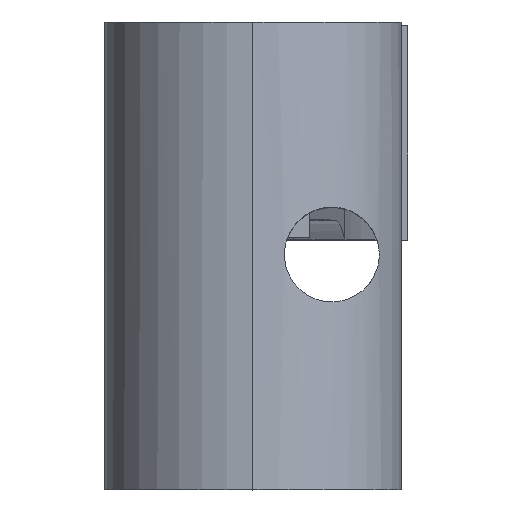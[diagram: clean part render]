
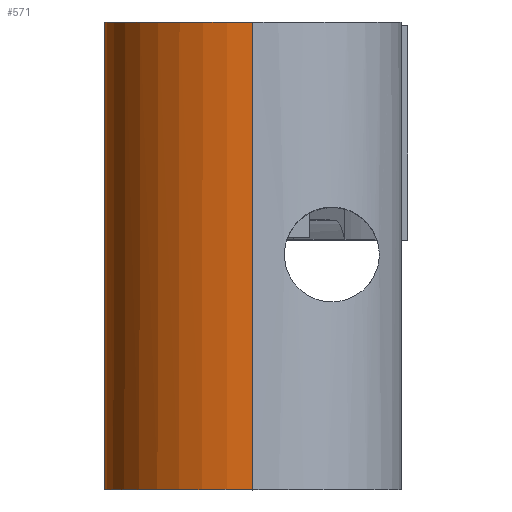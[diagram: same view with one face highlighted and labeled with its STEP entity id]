
A CAD part, top view. The second image highlights one B-rep face of the part: STEP entity #571.
In plain terms, the highlighted cylindrical face has radius 2.985 mm (diameter 5.969 mm), a partial arc.
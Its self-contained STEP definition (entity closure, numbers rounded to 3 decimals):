
#3 = CARTESIAN_POINT ( 'NONE',  ( 0., -4.318, 0. ) ) ;
#36 = ORIENTED_EDGE ( 'NONE', *, *, #305, .F. ) ;
#38 = ORIENTED_EDGE ( 'NONE', *, *, #936, .F. ) ;
#41 = ORIENTED_EDGE ( 'NONE', *, *, #340, .T. ) ;
#44 = CIRCLE ( 'NONE', #182, 2.985 ) ;
#50 = ORIENTED_EDGE ( 'NONE', *, *, #893, .F. ) ;
#61 = ORIENTED_EDGE ( 'NONE', *, *, #1059, .T. ) ;
#63 = VERTEX_POINT ( 'NONE', #675 ) ;
#82 = DIRECTION ( 'NONE',  ( 0., 0., 1. ) ) ;
#83 = EDGE_LOOP ( 'NONE', ( #36, #38, #504, #41, #50, #61 ) ) ;
#90 = LINE ( 'NONE', #626, #463 ) ;
#123 = CYLINDRICAL_SURFACE ( 'NONE', #316, 2.985 ) ;
#182 = AXIS2_PLACEMENT_3D ( 'NONE', #3, #647, #82 ) ;
#224 = AXIS2_PLACEMENT_3D ( 'NONE', #686, #684, #679 ) ;
#231 = VERTEX_POINT ( 'NONE', #1053 ) ;
#253 = VECTOR ( 'NONE', #876, 1000. ) ;
#274 = VERTEX_POINT ( 'NONE', #941 ) ;
#305 = EDGE_CURVE ( 'NONE', #231, #1132, #633, .T. ) ;
#316 = AXIS2_PLACEMENT_3D ( 'NONE', #1149, #761, #1146 ) ;
#340 = EDGE_CURVE ( 'NONE', #935, #63, #933, .T. ) ;
#463 = VECTOR ( 'NONE', #765, 1000. ) ;
#504 = ORIENTED_EDGE ( 'NONE', *, *, #619, .T. ) ;
#527 = FACE_OUTER_BOUND ( 'NONE', #83, .T. ) ;
#570 = DIRECTION ( 'NONE',  ( 0., 1., 0. ) ) ;
#571 = ADVANCED_FACE ( 'NONE', ( #527 ), #123, .T. ) ;
#610 = DIRECTION ( 'NONE',  ( 0., -1., 0. ) ) ;
#615 = CARTESIAN_POINT ( 'NONE',  ( 0., 0., 0. ) ) ;
#619 = EDGE_CURVE ( 'NONE', #274, #935, #90, .T. ) ;
#622 = DIRECTION ( 'NONE',  ( 0., 0., -1. ) ) ;
#626 = CARTESIAN_POINT ( 'NONE',  ( 0., -9.398, 2.985 ) ) ;
#633 = LINE ( 'NONE', #791, #948 ) ;
#647 = DIRECTION ( 'NONE',  ( 0., -1., 0. ) ) ;
#675 = CARTESIAN_POINT ( 'NONE',  ( -0.635, 0., -2.916 ) ) ;
#679 = DIRECTION ( 'NONE',  ( 0., 0., -1. ) ) ;
#684 = DIRECTION ( 'NONE',  ( 0., -1., 0. ) ) ;
#686 = CARTESIAN_POINT ( 'NONE',  ( 0., -9.398, 0. ) ) ;
#701 = AXIS2_PLACEMENT_3D ( 'NONE', #615, #610, #622 ) ;
#746 = CARTESIAN_POINT ( 'NONE',  ( 0., -4.318, -2.985 ) ) ;
#761 = DIRECTION ( 'NONE',  ( 0., 1., 0. ) ) ;
#765 = DIRECTION ( 'NONE',  ( 0., 1., 0. ) ) ;
#768 = CARTESIAN_POINT ( 'NONE',  ( 0., 0., 2.985 ) ) ;
#791 = CARTESIAN_POINT ( 'NONE',  ( 0., -9.398, -2.985 ) ) ;
#793 = LINE ( 'NONE', #880, #253 ) ;
#876 = DIRECTION ( 'NONE',  ( 0., 1., 0. ) ) ;
#880 = CARTESIAN_POINT ( 'NONE',  ( -0.635, -4.318, -2.916 ) ) ;
#893 = EDGE_CURVE ( 'NONE', #1046, #63, #793, .T. ) ;
#933 = CIRCLE ( 'NONE', #701, 2.985 ) ;
#935 = VERTEX_POINT ( 'NONE', #768 ) ;
#936 = EDGE_CURVE ( 'NONE', #274, #231, #1020, .T. ) ;
#941 = CARTESIAN_POINT ( 'NONE',  ( 0., -9.398, 2.985 ) ) ;
#948 = VECTOR ( 'NONE', #570, 1000. ) ;
#1020 = CIRCLE ( 'NONE', #224, 2.985 ) ;
#1046 = VERTEX_POINT ( 'NONE', #1175 ) ;
#1053 = CARTESIAN_POINT ( 'NONE',  ( 0., -9.398, -2.985 ) ) ;
#1059 = EDGE_CURVE ( 'NONE', #1046, #1132, #44, .T. ) ;
#1132 = VERTEX_POINT ( 'NONE', #746 ) ;
#1146 = DIRECTION ( 'NONE',  ( 0., 0., 1. ) ) ;
#1149 = CARTESIAN_POINT ( 'NONE',  ( 0., -9.398, 0. ) ) ;
#1175 = CARTESIAN_POINT ( 'NONE',  ( -0.635, -4.318, -2.916 ) ) ;
